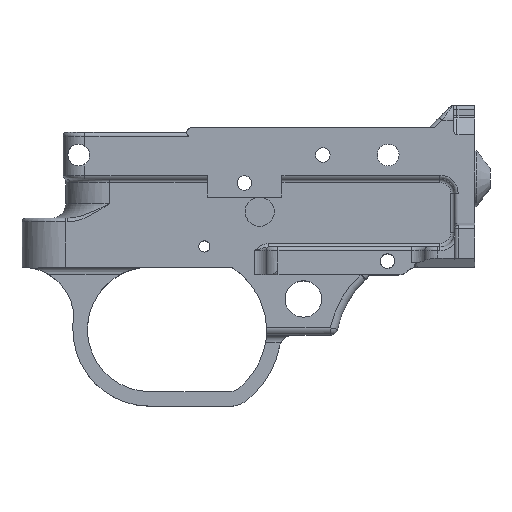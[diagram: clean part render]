
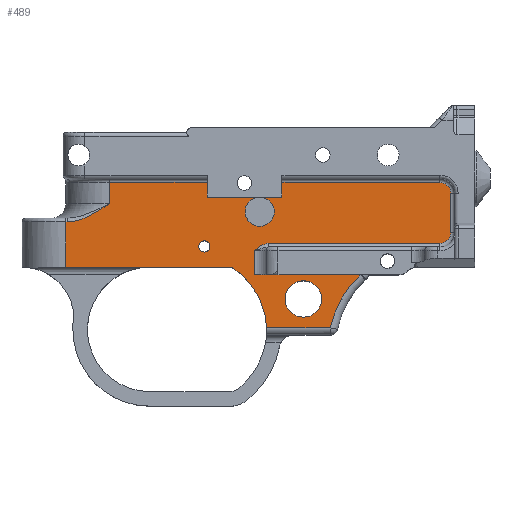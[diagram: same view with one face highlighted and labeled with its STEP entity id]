
A CAD part, top view. The second image highlights one B-rep face of the part: STEP entity #489.
In plain terms, the highlighted planar face has unit normal (0, 0, 1).
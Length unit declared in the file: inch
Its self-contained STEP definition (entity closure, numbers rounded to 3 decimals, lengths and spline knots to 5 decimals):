
#256=CARTESIAN_POINT('',(0.61891,0.17001,0.0275));
#257=VERTEX_POINT('',#256);
#258=CARTESIAN_POINT('',(0.61891,0.04501,0.0275));
#259=DIRECTION('',(0.0,0.0,-1.0));
#260=DIRECTION('',(-1.0,0.0,0.0));
#261=AXIS2_PLACEMENT_3D('',#258,#259,#260);
#262=CIRCLE('',#261,0.125);
#263=EDGE_CURVE('',#257,#257,#262,.T.);
#279=CARTESIAN_POINT('',(0.40372,0.03451,0.0275));
#280=DIRECTION('',(0.0,0.0,1.0));
#281=DIRECTION('',(1.0,0.0,0.0));
#282=AXIS2_PLACEMENT_3D('',#279,#280,#281);
#283=PLANE('',#282);
#284=CARTESIAN_POINT('',(0.57252,-0.28924,0.0275));
#285=VERTEX_POINT('',#284);
#286=CARTESIAN_POINT('',(0.57252,-0.49799,0.0275));
#287=VERTEX_POINT('',#286);
#288=CARTESIAN_POINT('',(0.57252,-0.28924,0.0275));
#289=DIRECTION('',(0.0,-1.0,0.0));
#290=VECTOR('',#289,0.20875);
#291=LINE('',#288,#290);
#292=EDGE_CURVE('',#285,#287,#291,.T.);
#293=ORIENTED_EDGE('',*,*,#292,.F.);
#294=CARTESIAN_POINT('',(0.69752,-0.22674,0.0275));
#295=VERTEX_POINT('',#294);
#296=CARTESIAN_POINT('',(0.69752,-0.22674,0.0275));
#297=CARTESIAN_POINT('',(0.67864,-0.22674,0.0275));
#298=CARTESIAN_POINT('',(0.65072,-0.23499,0.0275));
#299=CARTESIAN_POINT('',(0.61006,-0.25874,0.0275));
#300=CARTESIAN_POINT('',(0.58738,-0.27711,0.0275));
#301=CARTESIAN_POINT('',(0.57268,-0.28911,0.0275));
#302=CARTESIAN_POINT('',(0.5726,-0.28917,0.0275));
#303=CARTESIAN_POINT('',(0.57252,-0.28924,0.0275));
#304=B_SPLINE_CURVE_WITH_KNOTS('',3,(#296,#297,#298,#299,#300,#301,#302,#303),.UNSPECIFIED.,.F.,.U.,(4,1,1,2,4),(-0.35962,-0.21577,-0.14385,0.0,0.00076),.UNSPECIFIED.);
#305=EDGE_CURVE('',#295,#285,#304,.T.);
#306=ORIENTED_EDGE('',*,*,#305,.F.);
#307=CARTESIAN_POINT('',(2.16591,-0.22674,0.0275));
#308=VERTEX_POINT('',#307);
#309=CARTESIAN_POINT('',(2.16591,-0.22674,0.0275));
#310=DIRECTION('',(-1.0,0.0,0.0));
#311=VECTOR('',#310,1.46839);
#312=LINE('',#309,#311);
#313=EDGE_CURVE('',#308,#295,#312,.T.);
#314=ORIENTED_EDGE('',*,*,#313,.F.);
#315=CARTESIAN_POINT('',(2.25966,-0.13299,0.0275));
#316=VERTEX_POINT('',#315);
#317=CARTESIAN_POINT('',(2.16591,-0.13299,0.0275));
#318=DIRECTION('',(0.,0.,-1.0));
#319=DIRECTION('',(0.707,-0.707,0.));
#320=AXIS2_PLACEMENT_3D('',#317,#318,#319);
#321=CIRCLE('',#320,0.09375);
#322=EDGE_CURVE('',#316,#308,#321,.T.);
#323=ORIENTED_EDGE('',*,*,#322,.F.);
#324=CARTESIAN_POINT('',(2.25966,0.20201,0.0275));
#325=VERTEX_POINT('',#324);
#326=CARTESIAN_POINT('',(2.25966,0.20201,0.0275));
#327=DIRECTION('',(0.0,-1.0,0.0));
#328=VECTOR('',#327,0.335);
#329=LINE('',#326,#328);
#330=EDGE_CURVE('',#325,#316,#329,.T.);
#331=ORIENTED_EDGE('',*,*,#330,.F.);
#332=CARTESIAN_POINT('',(2.16591,0.29576,0.0275));
#333=VERTEX_POINT('',#332);
#334=CARTESIAN_POINT('',(2.16591,0.20201,0.0275));
#335=DIRECTION('',(0.,0.,-1.0));
#336=DIRECTION('',(0.707,0.707,0.));
#337=AXIS2_PLACEMENT_3D('',#334,#335,#336);
#338=CIRCLE('',#337,0.09375);
#339=EDGE_CURVE('',#333,#325,#338,.T.);
#340=ORIENTED_EDGE('',*,*,#339,.F.);
#341=CARTESIAN_POINT('',(0.81041,0.29576,0.0275));
#342=VERTEX_POINT('',#341);
#343=CARTESIAN_POINT('',(0.81041,0.29576,0.0275));
#344=DIRECTION('',(1.0,0.0,0.0));
#345=VECTOR('',#344,1.3555);
#346=LINE('',#343,#345);
#347=EDGE_CURVE('',#342,#333,#346,.T.);
#348=ORIENTED_EDGE('',*,*,#347,.F.);
#349=CARTESIAN_POINT('',(0.81041,0.17001,0.0275));
#350=VERTEX_POINT('',#349);
#351=CARTESIAN_POINT('',(0.81041,0.29576,0.0275));
#352=DIRECTION('',(0.0,-1.0,0.0));
#353=VECTOR('',#352,0.12575);
#354=LINE('',#351,#353);
#355=EDGE_CURVE('',#342,#350,#354,.T.);
#356=ORIENTED_EDGE('',*,*,#355,.T.);
#357=CARTESIAN_POINT('',(0.81041,0.17001,0.0275));
#358=DIRECTION('',(-1.0,0.0,0.0));
#359=VECTOR('',#358,0.1915);
#360=LINE('',#357,#359);
#361=EDGE_CURVE('',#350,#257,#360,.T.);
#362=ORIENTED_EDGE('',*,*,#361,.T.);
#363=ORIENTED_EDGE('',*,*,#263,.T.);
#364=CARTESIAN_POINT('',(0.16941,0.17001,0.0275));
#365=VERTEX_POINT('',#364);
#366=CARTESIAN_POINT('',(0.61891,0.17001,0.0275));
#367=DIRECTION('',(-1.0,0.0,0.0));
#368=VECTOR('',#367,0.4495);
#369=LINE('',#366,#368);
#370=EDGE_CURVE('',#257,#365,#369,.T.);
#371=ORIENTED_EDGE('',*,*,#370,.T.);
#372=CARTESIAN_POINT('',(0.16941,0.29576,0.0275));
#373=VERTEX_POINT('',#372);
#374=CARTESIAN_POINT('',(0.16941,0.17001,0.0275));
#375=DIRECTION('',(0.0,1.0,0.0));
#376=VECTOR('',#375,0.12575);
#377=LINE('',#374,#376);
#378=EDGE_CURVE('',#365,#373,#377,.T.);
#379=ORIENTED_EDGE('',*,*,#378,.T.);
#380=CARTESIAN_POINT('',(-0.67109,0.29576,0.0275));
#381=VERTEX_POINT('',#380);
#382=CARTESIAN_POINT('',(-0.67109,0.29576,0.0275));
#383=DIRECTION('',(1.0,0.0,0.0));
#384=VECTOR('',#383,0.8405);
#385=LINE('',#382,#384);
#386=EDGE_CURVE('',#381,#373,#385,.T.);
#387=ORIENTED_EDGE('',*,*,#386,.F.);
#388=CARTESIAN_POINT('',(-0.67109,0.11401,0.0275));
#389=VERTEX_POINT('',#388);
#390=CARTESIAN_POINT('',(-0.67109,0.11401,0.0275));
#391=DIRECTION('',(0.0,1.0,0.0));
#392=VECTOR('',#391,0.18175);
#393=LINE('',#390,#392);
#394=EDGE_CURVE('',#389,#381,#393,.T.);
#395=ORIENTED_EDGE('',*,*,#394,.F.);
#396=CARTESIAN_POINT('',(-1.03418,-0.04224,0.0275));
#397=VERTEX_POINT('',#396);
#398=CARTESIAN_POINT('',(-1.03418,-0.04224,0.0275));
#399=CARTESIAN_POINT('',(-0.98093,-0.04224,0.0275));
#400=CARTESIAN_POINT('',(-0.90162,-0.02088,0.0275));
#401=CARTESIAN_POINT('',(-0.78316,0.03857,0.0275));
#402=CARTESIAN_POINT('',(-0.71564,0.08397,0.0275));
#403=CARTESIAN_POINT('',(-0.67138,0.11382,0.0275));
#404=CARTESIAN_POINT('',(-0.67123,0.11392,0.0275));
#405=CARTESIAN_POINT('',(-0.67109,0.11401,0.0275));
#406=B_SPLINE_CURVE_WITH_KNOTS('',3,(#398,#399,#400,#401,#402,#403,#404,#405),.UNSPECIFIED.,.F.,.U.,(4,1,1,2,4),(0.0,0.40574,0.60861,1.01434,1.01566),.UNSPECIFIED.);
#407=EDGE_CURVE('',#397,#389,#406,.T.);
#408=ORIENTED_EDGE('',*,*,#407,.F.);
#409=CARTESIAN_POINT('',(-1.04617,-0.04224,0.0275));
#410=VERTEX_POINT('',#409);
#411=CARTESIAN_POINT('',(-1.04617,-0.04224,0.0275));
#412=DIRECTION('',(1.0,0.0,0.0));
#413=VECTOR('',#412,0.01198);
#414=LINE('',#411,#413);
#415=EDGE_CURVE('',#410,#397,#414,.T.);
#416=ORIENTED_EDGE('',*,*,#415,.F.);
#417=CARTESIAN_POINT('',(-1.04617,-0.43099,0.0275));
#418=VERTEX_POINT('',#417);
#419=CARTESIAN_POINT('',(-1.04617,-0.43099,0.0275));
#420=DIRECTION('',(0.0,1.0,0.0));
#421=VECTOR('',#420,0.38875);
#422=LINE('',#419,#421);
#423=EDGE_CURVE('',#418,#410,#422,.T.);
#424=ORIENTED_EDGE('',*,*,#423,.F.);
#425=CARTESIAN_POINT('',(0.37883,-0.43099,0.0275));
#426=VERTEX_POINT('',#425);
#427=CARTESIAN_POINT('',(0.37883,-0.43099,0.0275));
#428=DIRECTION('',(-1.0,0.0,0.0));
#429=VECTOR('',#428,1.425);
#430=LINE('',#427,#429);
#431=EDGE_CURVE('',#426,#418,#430,.T.);
#432=ORIENTED_EDGE('',*,*,#431,.F.);
#433=CARTESIAN_POINT('',(0.6777,-0.95149,0.0275));
#434=VERTEX_POINT('',#433);
#435=CARTESIAN_POINT('',(0.02585,-0.97972,0.0275));
#436=DIRECTION('',(0.,0.,1.));
#437=DIRECTION('',(0.999,-0.053,0.));
#438=AXIS2_PLACEMENT_3D('',#435,#436,#437);
#439=CIRCLE('',#438,0.65247);
#440=EDGE_CURVE('',#434,#426,#439,.T.);
#441=ORIENTED_EDGE('',*,*,#440,.F.);
#442=CARTESIAN_POINT('',(1.22519,-0.95149,0.0275));
#443=VERTEX_POINT('',#442);
#444=CARTESIAN_POINT('',(1.22519,-0.95149,0.0275));
#445=DIRECTION('',(-1.0,0.0,0.0));
#446=VECTOR('',#445,0.54749);
#447=LINE('',#444,#446);
#448=EDGE_CURVE('',#443,#434,#447,.T.);
#449=ORIENTED_EDGE('',*,*,#448,.F.);
#450=CARTESIAN_POINT('',(1.48031,-0.49799,0.0275));
#451=VERTEX_POINT('',#450);
#452=CARTESIAN_POINT('',(2.07759,-1.13251,0.0275));
#453=DIRECTION('',(0.,0.,1.));
#454=DIRECTION('',(-0.863,0.505,0.));
#455=AXIS2_PLACEMENT_3D('',#452,#453,#454);
#456=CIRCLE('',#455,0.87141);
#457=EDGE_CURVE('',#451,#443,#456,.T.);
#458=ORIENTED_EDGE('',*,*,#457,.F.);
#459=CARTESIAN_POINT('',(1.48031,-0.49799,0.0275));
#460=DIRECTION('',(-1.0,0.0,0.0));
#461=VECTOR('',#460,0.90779);
#462=LINE('',#459,#461);
#463=EDGE_CURVE('',#451,#287,#462,.T.);
#464=ORIENTED_EDGE('',*,*,#463,.T.);
#465=EDGE_LOOP('',(#293,#306,#314,#323,#331,#340,#348,#356,#362,#363,#371,#379,#387,#395,#408,#416,#424,#432,#441,#449,#458,#464));
#466=FACE_OUTER_BOUND('',#465,.T.);
#467=CARTESIAN_POINT('',(1.15016,-0.70399,0.0275));
#468=VERTEX_POINT('',#467);
#469=CARTESIAN_POINT('',(0.99391,-0.70399,0.0275));
#470=DIRECTION('',(0.0,0.0,-1.0));
#471=DIRECTION('',(-1.0,0.0,0.0));
#472=AXIS2_PLACEMENT_3D('',#469,#470,#471);
#473=CIRCLE('',#472,0.15625);
#474=EDGE_CURVE('',#468,#468,#473,.T.);
#475=ORIENTED_EDGE('',*,*,#474,.T.);
#476=EDGE_LOOP('',(#475));
#477=FACE_BOUND('',#476,.T.);
#478=CARTESIAN_POINT('',(0.19191,-0.25299,0.0275));
#479=VERTEX_POINT('',#478);
#480=CARTESIAN_POINT('',(0.14391,-0.25299,0.0275));
#481=DIRECTION('',(0.0,0.0,-1.0));
#482=DIRECTION('',(1.0,0.0,0.0));
#483=AXIS2_PLACEMENT_3D('',#480,#481,#482);
#484=CIRCLE('',#483,0.048);
#485=EDGE_CURVE('',#479,#479,#484,.T.);
#486=ORIENTED_EDGE('',*,*,#485,.T.);
#487=EDGE_LOOP('',(#486));
#488=FACE_BOUND('',#487,.T.);
#489=ADVANCED_FACE('',(#466,#477,#488),#283,.T.);
